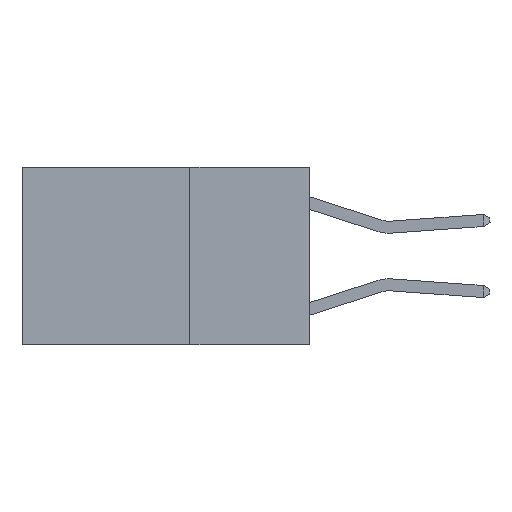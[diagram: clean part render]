
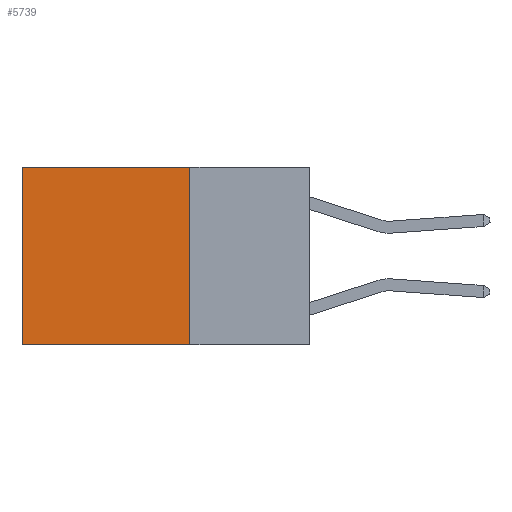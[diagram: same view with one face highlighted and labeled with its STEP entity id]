
A CAD part, left-side view. The second image highlights one B-rep face of the part: STEP entity #5739.
In plain terms, the highlighted planar face has unit normal (-1, 0, 0).
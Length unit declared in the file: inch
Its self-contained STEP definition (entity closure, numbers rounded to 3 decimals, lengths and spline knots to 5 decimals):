
#446 = VERTEX_POINT ( 'NONE', #1066 ) ;
#1066 = CARTESIAN_POINT ( 'NONE',  ( 0.2625, 0.6, -0.37 ) ) ;
#1422 = VECTOR ( 'NONE', #17470, 39.37008 ) ;
#1696 = EDGE_CURVE ( 'NONE', #4295, #446, #10454, .T. ) ;
#2199 = LINE ( 'NONE', #12338, #12229 ) ;
#2206 = ORIENTED_EDGE ( 'NONE', *, *, #10686, .F. ) ;
#2250 = CARTESIAN_POINT ( 'NONE',  ( 0.2625, 0.6, 0. ) ) ;
#3577 = DIRECTION ( 'NONE',  ( 1., 0., 0. ) ) ;
#3638 = DIRECTION ( 'NONE',  ( 0., 1., 0. ) ) ;
#4295 = VERTEX_POINT ( 'NONE', #15684 ) ;
#4499 = ORIENTED_EDGE ( 'NONE', *, *, #1696, .F. ) ;
#4633 = LINE ( 'NONE', #9353, #1422 ) ;
#5739 = ADVANCED_FACE ( 'NONE', ( #6492 ), #11680, .F. ) ;
#6040 = EDGE_CURVE ( 'NONE', #17311, #15785, #2199, .T. ) ;
#6492 = FACE_OUTER_BOUND ( 'NONE', #12434, .T. ) ;
#6500 = CARTESIAN_POINT ( 'NONE',  ( 0.2625, 0.25, 0. ) ) ;
#6841 = VECTOR ( 'NONE', #3638, 39.37008 ) ;
#8291 = DIRECTION ( 'NONE',  ( 0., 1., 0. ) ) ;
#9140 = VECTOR ( 'NONE', #13290, 39.37008 ) ;
#9353 = CARTESIAN_POINT ( 'NONE',  ( 0.2625, 0.6, 0. ) ) ;
#10447 = CARTESIAN_POINT ( 'NONE',  ( 0.2625, 0.25, -0.37 ) ) ;
#10454 = LINE ( 'NONE', #10447, #6841 ) ;
#10686 = EDGE_CURVE ( 'NONE', #17311, #4295, #16367, .T. ) ;
#11680 = PLANE ( 'NONE',  #12222 ) ;
#11740 = CARTESIAN_POINT ( 'NONE',  ( 0.2625, 0.25, 0. ) ) ;
#11938 = CARTESIAN_POINT ( 'NONE',  ( 0.2625, 0.25, 0. ) ) ;
#12222 = AXIS2_PLACEMENT_3D ( 'NONE', #11740, #3577, #13098 ) ;
#12229 = VECTOR ( 'NONE', #8291, 39.37008 ) ;
#12338 = CARTESIAN_POINT ( 'NONE',  ( 0.2625, 0.25, 0. ) ) ;
#12434 = EDGE_LOOP ( 'NONE', ( #13373, #4499, #2206, #12638 ) ) ;
#12638 = ORIENTED_EDGE ( 'NONE', *, *, #6040, .T. ) ;
#13098 = DIRECTION ( 'NONE',  ( 0., 0., -1. ) ) ;
#13290 = DIRECTION ( 'NONE',  ( 0., 0., -1. ) ) ;
#13373 = ORIENTED_EDGE ( 'NONE', *, *, #17397, .T. ) ;
#15684 = CARTESIAN_POINT ( 'NONE',  ( 0.2625, 0.25, -0.37 ) ) ;
#15785 = VERTEX_POINT ( 'NONE', #2250 ) ;
#16367 = LINE ( 'NONE', #11938, #9140 ) ;
#17311 = VERTEX_POINT ( 'NONE', #6500 ) ;
#17397 = EDGE_CURVE ( 'NONE', #15785, #446, #4633, .T. ) ;
#17470 = DIRECTION ( 'NONE',  ( 0., 0., -1. ) ) ;
